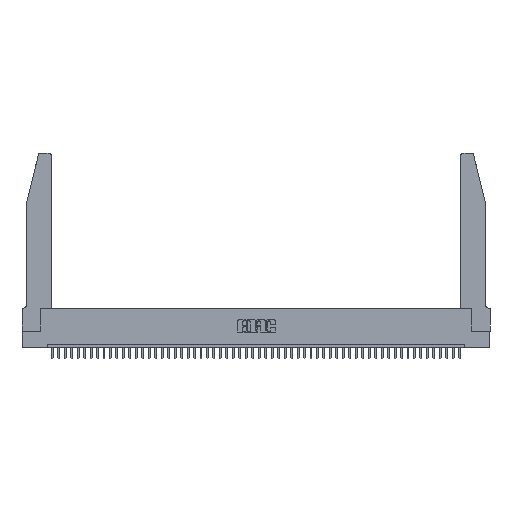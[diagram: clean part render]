
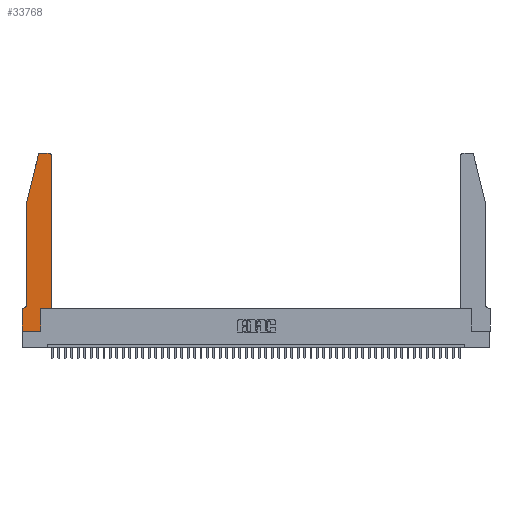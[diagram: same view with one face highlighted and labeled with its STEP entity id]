
A CAD part, top view. The second image highlights one B-rep face of the part: STEP entity #33768.
In plain terms, the highlighted planar face has unit normal (0, 0, 1).
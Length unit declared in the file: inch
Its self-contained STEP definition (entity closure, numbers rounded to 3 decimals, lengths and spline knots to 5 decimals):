
#34 = VERTEX_POINT ( 'NONE', #7103 ) ;
#556 = ORIENTED_EDGE ( 'NONE', *, *, #16938, .T. ) ;
#791 = FACE_OUTER_BOUND ( 'NONE', #22951, .T. ) ;
#877 = VERTEX_POINT ( 'NONE', #39019 ) ;
#1304 = DIRECTION ( 'NONE',  ( 0., 0., -1. ) ) ;
#1859 = CARTESIAN_POINT ( 'NONE',  ( 0.2865, 0., 0.37 ) ) ;
#3098 = VERTEX_POINT ( 'NONE', #4058 ) ;
#3486 = VERTEX_POINT ( 'NONE', #29008 ) ;
#4058 = CARTESIAN_POINT ( 'NONE',  ( 0.0755, 2., 0.37 ) ) ;
#4403 = LINE ( 'NONE', #24609, #36518 ) ;
#4931 = VECTOR ( 'NONE', #6005, 39.37008 ) ;
#5174 = DIRECTION ( 'NONE',  ( -1., 0., 0. ) ) ;
#5336 = LINE ( 'NONE', #18737, #14599 ) ;
#5521 = LINE ( 'NONE', #13360, #31512 ) ;
#6005 = DIRECTION ( 'NONE',  ( 1., 0., 0. ) ) ;
#6018 = VERTEX_POINT ( 'NONE', #20463 ) ;
#6636 = VERTEX_POINT ( 'NONE', #31469 ) ;
#7103 = CARTESIAN_POINT ( 'NONE',  ( 0.284, 2.75, 0.37 ) ) ;
#7758 = VERTEX_POINT ( 'NONE', #19707 ) ;
#7910 = VERTEX_POINT ( 'NONE', #46528 ) ;
#8157 = LINE ( 'NONE', #11706, #49382 ) ;
#9143 = ORIENTED_EDGE ( 'NONE', *, *, #36893, .T. ) ;
#9393 = DIRECTION ( 'NONE',  ( 0., -1., 0. ) ) ;
#9541 = CARTESIAN_POINT ( 'NONE',  ( 0.2865, 0.35, 0.37 ) ) ;
#10971 = ORIENTED_EDGE ( 'NONE', *, *, #30881, .T. ) ;
#11706 = CARTESIAN_POINT ( 'NONE',  ( 0.4505, 0.35, 0.37 ) ) ;
#13360 = CARTESIAN_POINT ( 'NONE',  ( 0.4505, 0.35, 0.37 ) ) ;
#13479 = AXIS2_PLACEMENT_3D ( 'NONE', #17662, #21215, #25098 ) ;
#14599 = VECTOR ( 'NONE', #22967, 39.37008 ) ;
#15125 = EDGE_CURVE ( 'NONE', #3486, #6018, #5336, .T. ) ;
#15332 = CARTESIAN_POINT ( 'NONE',  ( 0.4505, 0.35, 0.37 ) ) ;
#16364 = DIRECTION ( 'NONE',  ( -1., 0., 0. ) ) ;
#16495 = ORIENTED_EDGE ( 'NONE', *, *, #37389, .T. ) ;
#16938 = EDGE_CURVE ( 'NONE', #46869, #6636, #8157, .T. ) ;
#17300 = DIRECTION ( 'NONE',  ( 1., 0., 0. ) ) ;
#17662 = CARTESIAN_POINT ( 'NONE',  ( 0.4205, 2.72, 0.37 ) ) ;
#17776 = DIRECTION ( 'NONE',  ( -1., 0., 0. ) ) ;
#18307 = CARTESIAN_POINT ( 'NONE',  ( 0.2605, 2.75, 0.37 ) ) ;
#18737 = CARTESIAN_POINT ( 'NONE',  ( 0., 0., 0.37 ) ) ;
#18933 = VECTOR ( 'NONE', #5174, 39.37008 ) ;
#19707 = CARTESIAN_POINT ( 'NONE',  ( 0.4205, 2.75, 0.37 ) ) ;
#19760 = CIRCLE ( 'NONE', #36078, 0.03 ) ;
#20463 = CARTESIAN_POINT ( 'NONE',  ( 0., 0., 0.37 ) ) ;
#20860 = PLANE ( 'NONE',  #33600 ) ;
#21035 = DIRECTION ( 'NONE',  ( 0., 0., 1. ) ) ;
#21192 = ORIENTED_EDGE ( 'NONE', *, *, #26670, .T. ) ;
#21215 = DIRECTION ( 'NONE',  ( 0., 0., 1. ) ) ;
#21238 = CARTESIAN_POINT ( 'NONE',  ( 0.0055, 0.42, 0.37 ) ) ;
#21386 = VECTOR ( 'NONE', #17776, 39.37008 ) ;
#22723 = CARTESIAN_POINT ( 'NONE',  ( 0.0755, 2., 0.37 ) ) ;
#22951 = EDGE_LOOP ( 'NONE', ( #10971, #23988, #16495, #26801, #40758, #45555, #35916, #33743, #21192, #9143, #556, #42763 ) ) ;
#22956 = LINE ( 'NONE', #18307, #21386 ) ;
#22967 = DIRECTION ( 'NONE',  ( 0., -1., 0. ) ) ;
#23476 = EDGE_CURVE ( 'NONE', #3098, #877, #4403, .T. ) ;
#23636 = DIRECTION ( 'NONE',  ( -0.239, -0.971, 0. ) ) ;
#23988 = ORIENTED_EDGE ( 'NONE', *, *, #43309, .T. ) ;
#24435 = CARTESIAN_POINT ( 'NONE',  ( 0.0755, 0.35, 0.37 ) ) ;
#24544 = VERTEX_POINT ( 'NONE', #45432 ) ;
#24609 = CARTESIAN_POINT ( 'NONE',  ( 0.0755, 2., 0.37 ) ) ;
#25098 = DIRECTION ( 'NONE',  ( 1., 0., 0. ) ) ;
#25128 = CARTESIAN_POINT ( 'NONE',  ( 0.2865, 0.35, 0.37 ) ) ;
#25734 = DIRECTION ( 'NONE',  ( 0., 1., 0. ) ) ;
#26670 = EDGE_CURVE ( 'NONE', #45333, #29834, #33899, .T. ) ;
#26801 = ORIENTED_EDGE ( 'NONE', *, *, #23476, .T. ) ;
#27366 = EDGE_CURVE ( 'NONE', #877, #24544, #44722, .T. ) ;
#29008 = CARTESIAN_POINT ( 'NONE',  ( 0., 0.35, 0.37 ) ) ;
#29628 = DIRECTION ( 'NONE',  ( 0., 0., 1. ) ) ;
#29834 = VERTEX_POINT ( 'NONE', #25128 ) ;
#30100 = CARTESIAN_POINT ( 'NONE',  ( 0.284, 2.72, 0.37 ) ) ;
#30881 = EDGE_CURVE ( 'NONE', #7758, #34, #22956, .T. ) ;
#31469 = CARTESIAN_POINT ( 'NONE',  ( 0.4505, 2.72, 0.37 ) ) ;
#31478 = VECTOR ( 'NONE', #23636, 39.37008 ) ;
#31512 = VECTOR ( 'NONE', #36917, 39.37008 ) ;
#32062 = LINE ( 'NONE', #22723, #31478 ) ;
#32760 = LINE ( 'NONE', #32841, #4931 ) ;
#32841 = CARTESIAN_POINT ( 'NONE',  ( 0., 0., 0.37 ) ) ;
#33600 = AXIS2_PLACEMENT_3D ( 'NONE', #43831, #21035, #17300 ) ;
#33743 = ORIENTED_EDGE ( 'NONE', *, *, #35365, .T. ) ;
#33768 = ADVANCED_FACE ( 'NONE', ( #791 ), #20860, .T. ) ;
#33899 = LINE ( 'NONE', #9541, #36276 ) ;
#35094 = EDGE_CURVE ( 'NONE', #24544, #3486, #44308, .T. ) ;
#35313 = EDGE_CURVE ( 'NONE', #6636, #7758, #44942, .T. ) ;
#35365 = EDGE_CURVE ( 'NONE', #6018, #45333, #32760, .T. ) ;
#35916 = ORIENTED_EDGE ( 'NONE', *, *, #15125, .T. ) ;
#36078 = AXIS2_PLACEMENT_3D ( 'NONE', #30100, #29628, #40591 ) ;
#36276 = VECTOR ( 'NONE', #48262, 39.37008 ) ;
#36518 = VECTOR ( 'NONE', #9393, 39.37008 ) ;
#36893 = EDGE_CURVE ( 'NONE', #29834, #46869, #5521, .T. ) ;
#36917 = DIRECTION ( 'NONE',  ( 1., 0., 0. ) ) ;
#37389 = EDGE_CURVE ( 'NONE', #7910, #3098, #32062, .T. ) ;
#38322 = AXIS2_PLACEMENT_3D ( 'NONE', #21238, #1304, #16364 ) ;
#39019 = CARTESIAN_POINT ( 'NONE',  ( 0.0755, 0.42, 0.37 ) ) ;
#40591 = DIRECTION ( 'NONE',  ( 1., 0., 0. ) ) ;
#40758 = ORIENTED_EDGE ( 'NONE', *, *, #27366, .T. ) ;
#42763 = ORIENTED_EDGE ( 'NONE', *, *, #35313, .T. ) ;
#43309 = EDGE_CURVE ( 'NONE', #34, #7910, #19760, .T. ) ;
#43831 = CARTESIAN_POINT ( 'NONE',  ( 0., 0.35, 0.37 ) ) ;
#44308 = LINE ( 'NONE', #24435, #18933 ) ;
#44722 = CIRCLE ( 'NONE', #38322, 0.07 ) ;
#44942 = CIRCLE ( 'NONE', #13479, 0.03 ) ;
#45333 = VERTEX_POINT ( 'NONE', #1859 ) ;
#45432 = CARTESIAN_POINT ( 'NONE',  ( 0.0055, 0.35, 0.37 ) ) ;
#45555 = ORIENTED_EDGE ( 'NONE', *, *, #35094, .T. ) ;
#46528 = CARTESIAN_POINT ( 'NONE',  ( 0.25487, 2.72718, 0.37 ) ) ;
#46869 = VERTEX_POINT ( 'NONE', #15332 ) ;
#48262 = DIRECTION ( 'NONE',  ( 0., 1., 0. ) ) ;
#49382 = VECTOR ( 'NONE', #25734, 39.37008 ) ;
